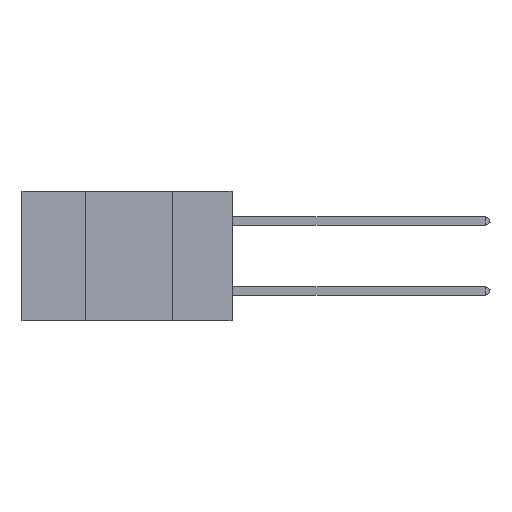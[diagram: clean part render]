
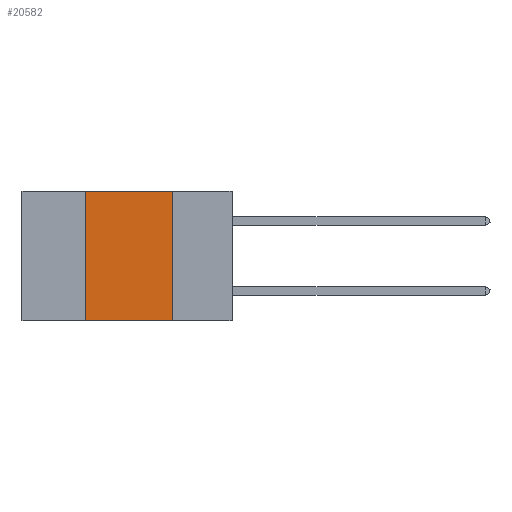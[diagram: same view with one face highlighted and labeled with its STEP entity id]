
A CAD part, left-side view. The second image highlights one B-rep face of the part: STEP entity #20582.
In plain terms, the highlighted planar face has unit normal (-1, 0, 0).
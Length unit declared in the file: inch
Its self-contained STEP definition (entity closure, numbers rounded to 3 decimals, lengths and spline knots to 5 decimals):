
#6 = LINE ( 'NONE', #223, #12926 ) ;
#221 = CARTESIAN_POINT ( 'NONE',  ( 0., 0.6, 0. ) ) ;
#223 = CARTESIAN_POINT ( 'NONE',  ( 0., 0.6, -0.37 ) ) ;
#1459 = VERTEX_POINT ( 'NONE', #9416 ) ;
#2276 = EDGE_CURVE ( 'NONE', #11230, #4163, #6, .T. ) ;
#2341 = CARTESIAN_POINT ( 'NONE',  ( 0., 0.17, 0. ) ) ;
#2975 = ORIENTED_EDGE ( 'NONE', *, *, #16204, .F. ) ;
#3436 = ORIENTED_EDGE ( 'NONE', *, *, #16351, .F. ) ;
#3626 = EDGE_LOOP ( 'NONE', ( #11874, #3436, #2975, #9657 ) ) ;
#4035 = DIRECTION ( 'NONE',  ( 0., 0., -1. ) ) ;
#4163 = VERTEX_POINT ( 'NONE', #4750 ) ;
#4750 = CARTESIAN_POINT ( 'NONE',  ( 0., 0.17, -0.37 ) ) ;
#4883 = DIRECTION ( 'NONE',  ( 0., 0., 1. ) ) ;
#5225 = VECTOR ( 'NONE', #4035, 39.37008 ) ;
#7366 = FACE_OUTER_BOUND ( 'NONE', #3626, .T. ) ;
#7694 = CARTESIAN_POINT ( 'NONE',  ( 0., 0.6, 0. ) ) ;
#8089 = VECTOR ( 'NONE', #4883, 39.37008 ) ;
#8351 = AXIS2_PLACEMENT_3D ( 'NONE', #7694, #18658, #9291 ) ;
#8456 = CARTESIAN_POINT ( 'NONE',  ( 0., 0.42, 0. ) ) ;
#8933 = VERTEX_POINT ( 'NONE', #8456 ) ;
#9291 = DIRECTION ( 'NONE',  ( 0., 0., -1. ) ) ;
#9416 = CARTESIAN_POINT ( 'NONE',  ( 0., 0.17, 0. ) ) ;
#9657 = ORIENTED_EDGE ( 'NONE', *, *, #2276, .T. ) ;
#11230 = VERTEX_POINT ( 'NONE', #14434 ) ;
#11874 = ORIENTED_EDGE ( 'NONE', *, *, #14471, .F. ) ;
#12248 = LINE ( 'NONE', #17481, #8089 ) ;
#12926 = VECTOR ( 'NONE', #14654, 39.37008 ) ;
#13967 = LINE ( 'NONE', #221, #14956 ) ;
#14434 = CARTESIAN_POINT ( 'NONE',  ( 0., 0.42, -0.37 ) ) ;
#14471 = EDGE_CURVE ( 'NONE', #1459, #4163, #18307, .T. ) ;
#14654 = DIRECTION ( 'NONE',  ( 0., -1., 0. ) ) ;
#14956 = VECTOR ( 'NONE', #17809, 39.37008 ) ;
#15528 = PLANE ( 'NONE',  #8351 ) ;
#16204 = EDGE_CURVE ( 'NONE', #11230, #8933, #12248, .T. ) ;
#16351 = EDGE_CURVE ( 'NONE', #8933, #1459, #13967, .T. ) ;
#17481 = CARTESIAN_POINT ( 'NONE',  ( 0., 0.42, 0. ) ) ;
#17809 = DIRECTION ( 'NONE',  ( 0., -1., 0. ) ) ;
#18307 = LINE ( 'NONE', #2341, #5225 ) ;
#18658 = DIRECTION ( 'NONE',  ( 1., 0., 0. ) ) ;
#20582 = ADVANCED_FACE ( 'NONE', ( #7366 ), #15528, .F. ) ;
